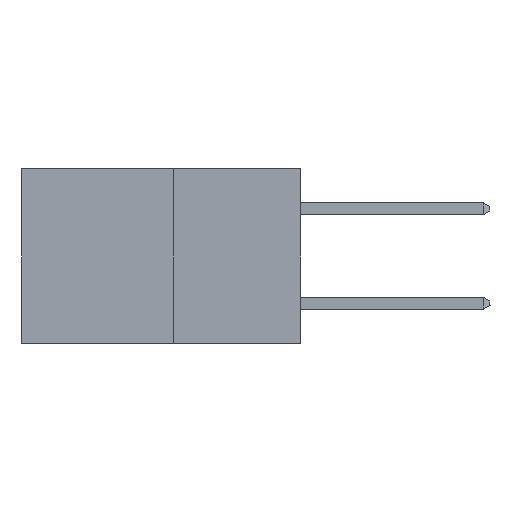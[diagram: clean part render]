
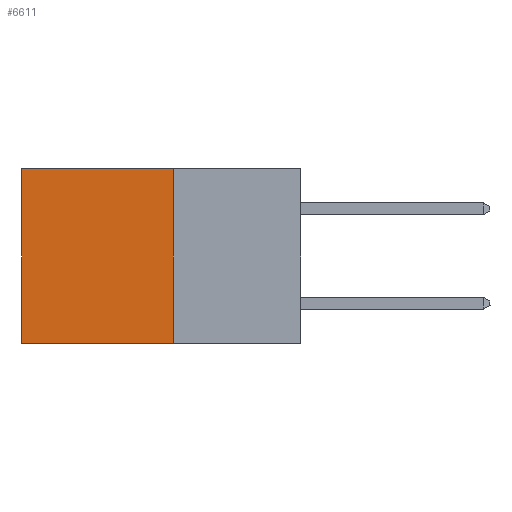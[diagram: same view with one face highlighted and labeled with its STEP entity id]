
A CAD part, left-side view. The second image highlights one B-rep face of the part: STEP entity #6611.
In plain terms, the highlighted planar face has unit normal (-1, 0, 0).
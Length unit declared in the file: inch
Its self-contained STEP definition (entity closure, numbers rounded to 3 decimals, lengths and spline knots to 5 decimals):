
#93 = CARTESIAN_POINT ( 'NONE',  ( 0.277, 0.59, 0. ) ) ;
#431 = VERTEX_POINT ( 'NONE', #25521 ) ;
#1694 = ORIENTED_EDGE ( 'NONE', *, *, #17923, .T. ) ;
#3031 = VERTEX_POINT ( 'NONE', #93 ) ;
#3397 = CARTESIAN_POINT ( 'NONE',  ( 0.277, 0.27, 0. ) ) ;
#4099 = VERTEX_POINT ( 'NONE', #21353 ) ;
#4758 = ORIENTED_EDGE ( 'NONE', *, *, #20338, .F. ) ;
#6422 = CARTESIAN_POINT ( 'NONE',  ( 0.277, 0.27, -0.37 ) ) ;
#6611 = ADVANCED_FACE ( 'NONE', ( #22448 ), #19190, .F. ) ;
#6811 = LINE ( 'NONE', #10184, #17701 ) ;
#6908 = VECTOR ( 'NONE', #24027, 39.37008 ) ;
#8402 = CARTESIAN_POINT ( 'NONE',  ( 0.277, 0.27, -0.37 ) ) ;
#9214 = AXIS2_PLACEMENT_3D ( 'NONE', #8402, #23477, #10586 ) ;
#10184 = CARTESIAN_POINT ( 'NONE',  ( 0.277, 0.27, -0.37 ) ) ;
#10586 = DIRECTION ( 'NONE',  ( 0., 0., -1. ) ) ;
#12367 = DIRECTION ( 'NONE',  ( 0., 1., 0. ) ) ;
#14928 = VECTOR ( 'NONE', #15115, 39.37008 ) ;
#15115 = DIRECTION ( 'NONE',  ( 0., 0., -1. ) ) ;
#15324 = EDGE_CURVE ( 'NONE', #18871, #4099, #21295, .T. ) ;
#16148 = ORIENTED_EDGE ( 'NONE', *, *, #15324, .F. ) ;
#16490 = VECTOR ( 'NONE', #23033, 39.37008 ) ;
#17701 = VECTOR ( 'NONE', #12367, 39.37008 ) ;
#17923 = EDGE_CURVE ( 'NONE', #3031, #431, #23486, .T. ) ;
#18582 = CARTESIAN_POINT ( 'NONE',  ( 0.277, 0.27, 0. ) ) ;
#18871 = VERTEX_POINT ( 'NONE', #18582 ) ;
#19190 = PLANE ( 'NONE',  #9214 ) ;
#20338 = EDGE_CURVE ( 'NONE', #4099, #431, #6811, .T. ) ;
#20914 = EDGE_LOOP ( 'NONE', ( #1694, #4758, #16148, #23343 ) ) ;
#21295 = LINE ( 'NONE', #6422, #14928 ) ;
#21353 = CARTESIAN_POINT ( 'NONE',  ( 0.277, 0.27, -0.37 ) ) ;
#21914 = CARTESIAN_POINT ( 'NONE',  ( 0.277, 0.59, -0.37 ) ) ;
#22448 = FACE_OUTER_BOUND ( 'NONE', #20914, .T. ) ;
#22850 = LINE ( 'NONE', #3397, #16490 ) ;
#23033 = DIRECTION ( 'NONE',  ( 0., 1., 0. ) ) ;
#23343 = ORIENTED_EDGE ( 'NONE', *, *, #24649, .T. ) ;
#23477 = DIRECTION ( 'NONE',  ( 1., 0., 0. ) ) ;
#23486 = LINE ( 'NONE', #21914, #6908 ) ;
#24027 = DIRECTION ( 'NONE',  ( 0., 0., -1. ) ) ;
#24649 = EDGE_CURVE ( 'NONE', #18871, #3031, #22850, .T. ) ;
#25521 = CARTESIAN_POINT ( 'NONE',  ( 0.277, 0.59, -0.37 ) ) ;
